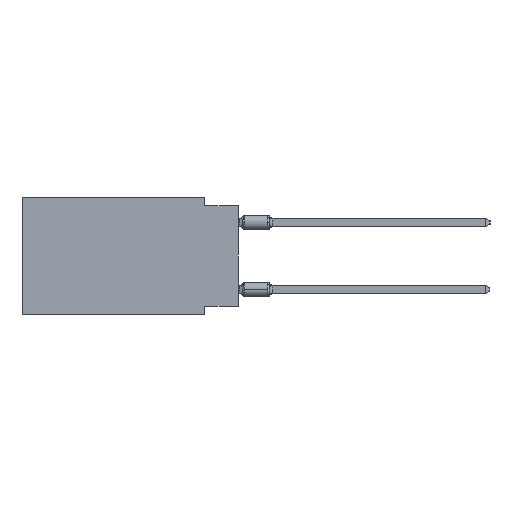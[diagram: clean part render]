
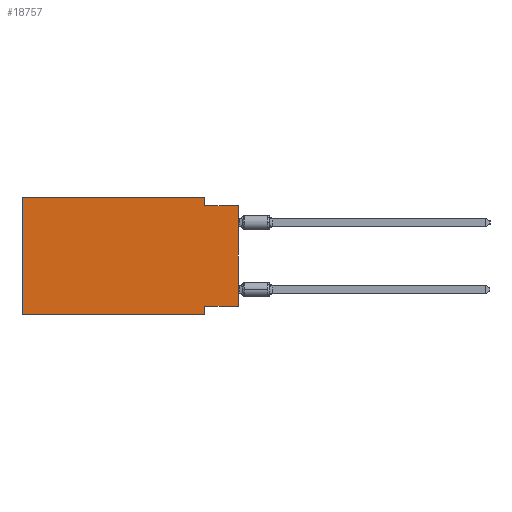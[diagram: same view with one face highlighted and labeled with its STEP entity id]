
A CAD part, left-side view. The second image highlights one B-rep face of the part: STEP entity #18757.
In plain terms, the highlighted planar face has unit normal (-1, 0, 0).
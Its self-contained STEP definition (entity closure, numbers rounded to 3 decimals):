
#15 = DIRECTION ( 'NONE',  ( 0., 0., 1. ) ) ;
#478 = CARTESIAN_POINT ( 'NONE',  ( 0., 16.383, 0. ) ) ;
#2140 = VERTEX_POINT ( 'NONE', #15711 ) ;
#2157 = DIRECTION ( 'NONE',  ( 1., 0., 0. ) ) ;
#2751 = CARTESIAN_POINT ( 'NONE',  ( 0., 2.54, 0. ) ) ;
#3727 = DIRECTION ( 'NONE',  ( 0., -1., 0. ) ) ;
#4364 = CARTESIAN_POINT ( 'NONE',  ( 0., 2.54, -8.89 ) ) ;
#4436 = VERTEX_POINT ( 'NONE', #2751 ) ;
#4555 = CARTESIAN_POINT ( 'NONE',  ( 0., 2.54, 0. ) ) ;
#4717 = LINE ( 'NONE', #14749, #24627 ) ;
#4778 = ORIENTED_EDGE ( 'NONE', *, *, #15128, .F. ) ;
#4795 = EDGE_CURVE ( 'NONE', #11497, #31582, #4717, .T. ) ;
#5095 = AXIS2_PLACEMENT_3D ( 'NONE', #6939, #2157, #16975 ) ;
#5139 = DIRECTION ( 'NONE',  ( 0., -1., 0. ) ) ;
#5305 = DIRECTION ( 'NONE',  ( 0., 0., -1. ) ) ;
#5345 = ORIENTED_EDGE ( 'NONE', *, *, #16870, .F. ) ;
#5621 = VECTOR ( 'NONE', #19104, 1000. ) ;
#6128 = EDGE_CURVE ( 'NONE', #6671, #18936, #22600, .T. ) ;
#6671 = VERTEX_POINT ( 'NONE', #19484 ) ;
#6769 = ORIENTED_EDGE ( 'NONE', *, *, #6884, .F. ) ;
#6884 = EDGE_CURVE ( 'NONE', #8395, #31582, #15674, .T. ) ;
#6939 = CARTESIAN_POINT ( 'NONE',  ( 0., 16.383, 0. ) ) ;
#7074 = EDGE_CURVE ( 'NONE', #11497, #2140, #26038, .T. ) ;
#7221 = VECTOR ( 'NONE', #5139, 1000. ) ;
#7558 = VECTOR ( 'NONE', #28950, 1000. ) ;
#8118 = EDGE_CURVE ( 'NONE', #2140, #29960, #17979, .T. ) ;
#8395 = VERTEX_POINT ( 'NONE', #31872 ) ;
#8743 = VECTOR ( 'NONE', #15, 1000. ) ;
#9006 = LINE ( 'NONE', #16559, #25505 ) ;
#9427 = PLANE ( 'NONE',  #5095 ) ;
#9837 = DIRECTION ( 'NONE',  ( 0., 0., -1. ) ) ;
#11330 = LINE ( 'NONE', #31422, #7558 ) ;
#11497 = VERTEX_POINT ( 'NONE', #27713 ) ;
#12708 = ORIENTED_EDGE ( 'NONE', *, *, #7074, .F. ) ;
#12737 = CARTESIAN_POINT ( 'NONE',  ( 0., 0., -0.635 ) ) ;
#13475 = EDGE_LOOP ( 'NONE', ( #24737, #6769, #5345, #4778, #29828, #15327, #19309, #12708 ) ) ;
#13540 = CARTESIAN_POINT ( 'NONE',  ( 0., 0., -8.255 ) ) ;
#14526 = CARTESIAN_POINT ( 'NONE',  ( 0., 16.383, 0. ) ) ;
#14667 = FACE_OUTER_BOUND ( 'NONE', #13475, .T. ) ;
#14749 = CARTESIAN_POINT ( 'NONE',  ( 0., 0., 0. ) ) ;
#15128 = EDGE_CURVE ( 'NONE', #18936, #4436, #11330, .T. ) ;
#15327 = ORIENTED_EDGE ( 'NONE', *, *, #21043, .T. ) ;
#15674 = LINE ( 'NONE', #25724, #7221 ) ;
#15711 = CARTESIAN_POINT ( 'NONE',  ( 0., 2.54, -8.255 ) ) ;
#16559 = CARTESIAN_POINT ( 'NONE',  ( 0., 16.383, -8.89 ) ) ;
#16870 = EDGE_CURVE ( 'NONE', #4436, #8395, #21852, .T. ) ;
#16975 = DIRECTION ( 'NONE',  ( 0., 0., -1. ) ) ;
#17979 = LINE ( 'NONE', #23255, #18817 ) ;
#18757 = ADVANCED_FACE ( 'NONE', ( #14667 ), #9427, .F. ) ;
#18817 = VECTOR ( 'NONE', #5305, 1000. ) ;
#18936 = VERTEX_POINT ( 'NONE', #478 ) ;
#19104 = DIRECTION ( 'NONE',  ( 0., 1., 0. ) ) ;
#19309 = ORIENTED_EDGE ( 'NONE', *, *, #8118, .F. ) ;
#19484 = CARTESIAN_POINT ( 'NONE',  ( 0., 16.383, -8.89 ) ) ;
#21043 = EDGE_CURVE ( 'NONE', #6671, #29960, #9006, .T. ) ;
#21852 = LINE ( 'NONE', #4555, #29730 ) ;
#22600 = LINE ( 'NONE', #14526, #8743 ) ;
#23255 = CARTESIAN_POINT ( 'NONE',  ( 0., 2.54, -8.89 ) ) ;
#24627 = VECTOR ( 'NONE', #24803, 1000. ) ;
#24737 = ORIENTED_EDGE ( 'NONE', *, *, #4795, .T. ) ;
#24803 = DIRECTION ( 'NONE',  ( 0., 0., 1. ) ) ;
#25505 = VECTOR ( 'NONE', #3727, 1000. ) ;
#25724 = CARTESIAN_POINT ( 'NONE',  ( 0., 0., -0.635 ) ) ;
#26038 = LINE ( 'NONE', #13540, #5621 ) ;
#27713 = CARTESIAN_POINT ( 'NONE',  ( 0., 0., -8.255 ) ) ;
#28950 = DIRECTION ( 'NONE',  ( 0., -1., 0. ) ) ;
#29730 = VECTOR ( 'NONE', #9837, 1000. ) ;
#29828 = ORIENTED_EDGE ( 'NONE', *, *, #6128, .F. ) ;
#29960 = VERTEX_POINT ( 'NONE', #4364 ) ;
#31422 = CARTESIAN_POINT ( 'NONE',  ( 0., 16.383, 0. ) ) ;
#31582 = VERTEX_POINT ( 'NONE', #12737 ) ;
#31872 = CARTESIAN_POINT ( 'NONE',  ( 0., 2.54, -0.635 ) ) ;
